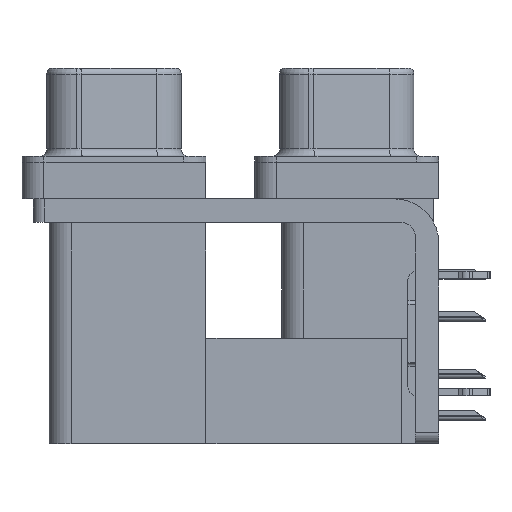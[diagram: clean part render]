
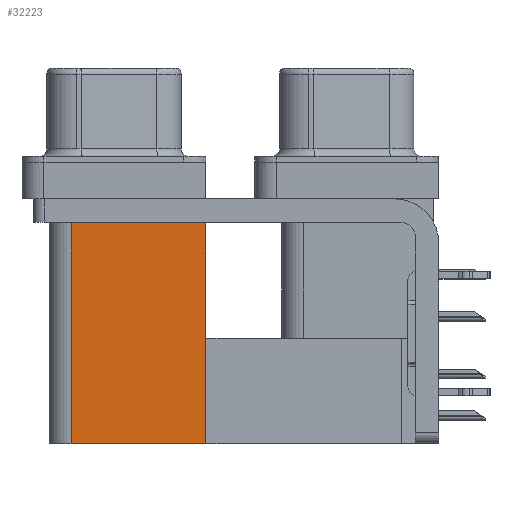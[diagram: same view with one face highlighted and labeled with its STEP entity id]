
A CAD part, left-side view. The second image highlights one B-rep face of the part: STEP entity #32223.
In plain terms, the highlighted planar face has unit normal (-1, 0, 0).
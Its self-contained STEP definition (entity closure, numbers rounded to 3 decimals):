
#7 = ORIENTED_EDGE ( 'NONE', *, *, #9797, .F. ) ;
#4613 = EDGE_CURVE ( 'NONE', #12192, #33975, #32414, .T. ) ;
#5140 = VECTOR ( 'NONE', #22605, 1000. ) ;
#7209 = DIRECTION ( 'NONE',  ( 0., 1., 0. ) ) ;
#9319 = CARTESIAN_POINT ( 'NONE',  ( 3.7, 18.8, -19.2 ) ) ;
#9797 = EDGE_CURVE ( 'NONE', #38309, #33975, #38399, .T. ) ;
#10513 = AXIS2_PLACEMENT_3D ( 'NONE', #40288, #15684, #33727 ) ;
#11227 = CARTESIAN_POINT ( 'NONE',  ( 3.7, 9.6, -19.2 ) ) ;
#12079 = LINE ( 'NONE', #37085, #13010 ) ;
#12192 = VERTEX_POINT ( 'NONE', #39654 ) ;
#12206 = FACE_OUTER_BOUND ( 'NONE', #38920, .T. ) ;
#13010 = VECTOR ( 'NONE', #21707, 1000. ) ;
#14265 = VECTOR ( 'NONE', #7209, 1000. ) ;
#15684 = DIRECTION ( 'NONE',  ( 1., 0., 0. ) ) ;
#16670 = CARTESIAN_POINT ( 'NONE',  ( 3.7, 18.8, -19.2 ) ) ;
#19635 = DIRECTION ( 'NONE',  ( 0., 0., 1. ) ) ;
#20101 = CARTESIAN_POINT ( 'NONE',  ( 3.7, 9.6, -2.5 ) ) ;
#20720 = EDGE_CURVE ( 'NONE', #26071, #12192, #35419, .T. ) ;
#21179 = ORIENTED_EDGE ( 'NONE', *, *, #20720, .T. ) ;
#21208 = PLANE ( 'NONE',  #10513 ) ;
#21707 = DIRECTION ( 'NONE',  ( 0., 1., 0. ) ) ;
#22605 = DIRECTION ( 'NONE',  ( 0., 0., 1. ) ) ;
#23551 = CARTESIAN_POINT ( 'NONE',  ( 3.7, 18.8, -2.5 ) ) ;
#24378 = CARTESIAN_POINT ( 'NONE',  ( 3.7, 9.6, -19.2 ) ) ;
#25630 = ORIENTED_EDGE ( 'NONE', *, *, #4613, .T. ) ;
#26071 = VERTEX_POINT ( 'NONE', #24378 ) ;
#30878 = ORIENTED_EDGE ( 'NONE', *, *, #37493, .F. ) ;
#31791 = VECTOR ( 'NONE', #19635, 1000. ) ;
#32223 = ADVANCED_FACE ( 'NONE', ( #12206 ), #21208, .F. ) ;
#32414 = LINE ( 'NONE', #20101, #14265 ) ;
#33727 = DIRECTION ( 'NONE',  ( 0., 0., -1. ) ) ;
#33975 = VERTEX_POINT ( 'NONE', #23551 ) ;
#35419 = LINE ( 'NONE', #11227, #31791 ) ;
#37085 = CARTESIAN_POINT ( 'NONE',  ( 3.7, 9.6, -19.2 ) ) ;
#37493 = EDGE_CURVE ( 'NONE', #26071, #38309, #12079, .T. ) ;
#38309 = VERTEX_POINT ( 'NONE', #9319 ) ;
#38399 = LINE ( 'NONE', #16670, #5140 ) ;
#38920 = EDGE_LOOP ( 'NONE', ( #25630, #7, #30878, #21179 ) ) ;
#39654 = CARTESIAN_POINT ( 'NONE',  ( 3.7, 9.6, -2.5 ) ) ;
#40288 = CARTESIAN_POINT ( 'NONE',  ( 3.7, 9.6, -19.2 ) ) ;
